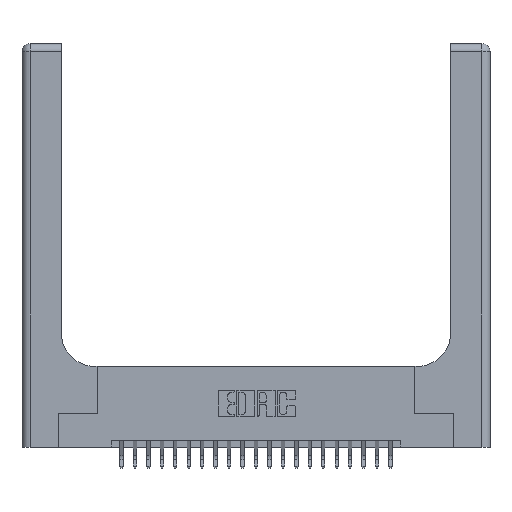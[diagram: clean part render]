
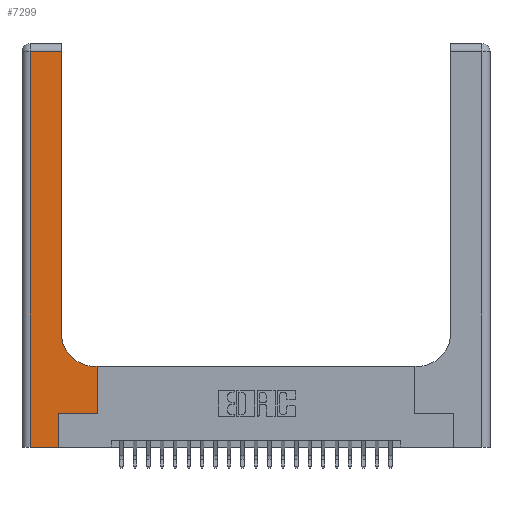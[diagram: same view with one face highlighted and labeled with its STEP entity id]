
A CAD part, top view. The second image highlights one B-rep face of the part: STEP entity #7299.
In plain terms, the highlighted planar face has unit normal (0, 0, 1).
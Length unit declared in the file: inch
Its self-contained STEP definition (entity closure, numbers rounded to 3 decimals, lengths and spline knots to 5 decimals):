
#592 = CARTESIAN_POINT ( 'NONE',  ( 0.269, 0.25, 0.37 ) ) ;
#1023 = VERTEX_POINT ( 'NONE', #11029 ) ;
#1548 = LINE ( 'NONE', #2361, #16248 ) ;
#1916 = VECTOR ( 'NONE', #7862, 39.37008 ) ;
#2361 = CARTESIAN_POINT ( 'NONE',  ( 0.06, 3., 0.37 ) ) ;
#2403 = VECTOR ( 'NONE', #12728, 39.37008 ) ;
#2799 = ORIENTED_EDGE ( 'NONE', *, *, #6019, .T. ) ;
#3022 = EDGE_CURVE ( 'NONE', #11211, #14283, #4676, .T. ) ;
#3046 = LINE ( 'NONE', #18708, #22686 ) ;
#3532 = CARTESIAN_POINT ( 'NONE',  ( 0.5585, 0.25, 0.37 ) ) ;
#3635 = CARTESIAN_POINT ( 'NONE',  ( 0., 3., 0.37 ) ) ;
#4118 = VERTEX_POINT ( 'NONE', #592 ) ;
#4665 = CIRCLE ( 'NONE', #6850, 0.25 ) ;
#4676 = LINE ( 'NONE', #8454, #23669 ) ;
#4746 = ORIENTED_EDGE ( 'NONE', *, *, #21546, .T. ) ;
#4850 = CARTESIAN_POINT ( 'NONE',  ( 0.2915, 2.94, 0.37 ) ) ;
#5420 = VERTEX_POINT ( 'NONE', #18527 ) ;
#5477 = DIRECTION ( 'NONE',  ( 0., 0., -1. ) ) ;
#5487 = DIRECTION ( 'NONE',  ( 0., 1., 0. ) ) ;
#5538 = DIRECTION ( 'NONE',  ( 1., 0., 0. ) ) ;
#5591 = DIRECTION ( 'NONE',  ( 0., 0., -1. ) ) ;
#5747 = VECTOR ( 'NONE', #5538, 39.37008 ) ;
#5763 = LINE ( 'NONE', #3532, #15256 ) ;
#5839 = ORIENTED_EDGE ( 'NONE', *, *, #22563, .T. ) ;
#6015 = FACE_OUTER_BOUND ( 'NONE', #13664, .T. ) ;
#6019 = EDGE_CURVE ( 'NONE', #18812, #18891, #17633, .T. ) ;
#6559 = CARTESIAN_POINT ( 'NONE',  ( 0.2915, 0.85, 0.37 ) ) ;
#6648 = EDGE_CURVE ( 'NONE', #4118, #5420, #10208, .T. ) ;
#6850 = AXIS2_PLACEMENT_3D ( 'NONE', #16830, #5477, #18752 ) ;
#7299 = ADVANCED_FACE ( 'NONE', ( #6015 ), #16934, .F. ) ;
#7862 = DIRECTION ( 'NONE',  ( 1., 0., 0. ) ) ;
#8205 = ORIENTED_EDGE ( 'NONE', *, *, #6648, .T. ) ;
#8454 = CARTESIAN_POINT ( 'NONE',  ( 0.2915, 0.6, 0.37 ) ) ;
#8519 = DIRECTION ( 'NONE',  ( 0., 1., 0. ) ) ;
#8708 = VERTEX_POINT ( 'NONE', #9640 ) ;
#9268 = VECTOR ( 'NONE', #8519, 39.37008 ) ;
#9473 = EDGE_CURVE ( 'NONE', #17769, #4118, #10453, .T. ) ;
#9640 = CARTESIAN_POINT ( 'NONE',  ( 0.06, 0., 0.37 ) ) ;
#10208 = LINE ( 'NONE', #18807, #5747 ) ;
#10453 = LINE ( 'NONE', #21782, #9268 ) ;
#11029 = CARTESIAN_POINT ( 'NONE',  ( 0.06, 2.94, 0.37 ) ) ;
#11211 = VERTEX_POINT ( 'NONE', #21859 ) ;
#11265 = ORIENTED_EDGE ( 'NONE', *, *, #9473, .T. ) ;
#12324 = CARTESIAN_POINT ( 'NONE',  ( 0.269, 0., 0.37 ) ) ;
#12728 = DIRECTION ( 'NONE',  ( 0., 1., 0. ) ) ;
#13084 = DIRECTION ( 'NONE',  ( -1., 0., 0. ) ) ;
#13664 = EDGE_LOOP ( 'NONE', ( #2799, #16541, #21298, #4746, #11265, #8205, #18872, #24474, #5839 ) ) ;
#13856 = DIRECTION ( 'NONE',  ( 0., -1., 0. ) ) ;
#14174 = EDGE_CURVE ( 'NONE', #18891, #1023, #3046, .T. ) ;
#14283 = VERTEX_POINT ( 'NONE', #21269 ) ;
#14622 = CARTESIAN_POINT ( 'NONE',  ( 0.2915, 3., 0.37 ) ) ;
#14730 = EDGE_CURVE ( 'NONE', #5420, #11211, #5763, .T. ) ;
#15256 = VECTOR ( 'NONE', #5487, 39.37008 ) ;
#15473 = CARTESIAN_POINT ( 'NONE',  ( 0., 0., 0.37 ) ) ;
#16248 = VECTOR ( 'NONE', #13856, 39.37008 ) ;
#16541 = ORIENTED_EDGE ( 'NONE', *, *, #14174, .T. ) ;
#16830 = CARTESIAN_POINT ( 'NONE',  ( 0.5415, 0.85, 0.37 ) ) ;
#16934 = PLANE ( 'NONE',  #20056 ) ;
#17633 = LINE ( 'NONE', #14622, #2403 ) ;
#17769 = VERTEX_POINT ( 'NONE', #12324 ) ;
#17786 = LINE ( 'NONE', #15473, #1916 ) ;
#18527 = CARTESIAN_POINT ( 'NONE',  ( 0.5585, 0.25, 0.37 ) ) ;
#18708 = CARTESIAN_POINT ( 'NONE',  ( 0., 2.94, 0.37 ) ) ;
#18752 = DIRECTION ( 'NONE',  ( 1., 0., 0. ) ) ;
#18807 = CARTESIAN_POINT ( 'NONE',  ( 0.269, 0.25, 0.37 ) ) ;
#18812 = VERTEX_POINT ( 'NONE', #6559 ) ;
#18855 = DIRECTION ( 'NONE',  ( -1., 0., 0. ) ) ;
#18872 = ORIENTED_EDGE ( 'NONE', *, *, #14730, .T. ) ;
#18891 = VERTEX_POINT ( 'NONE', #4850 ) ;
#20056 = AXIS2_PLACEMENT_3D ( 'NONE', #3635, #5591, #18855 ) ;
#20499 = EDGE_CURVE ( 'NONE', #1023, #8708, #1548, .T. ) ;
#21269 = CARTESIAN_POINT ( 'NONE',  ( 0.5415, 0.6, 0.37 ) ) ;
#21298 = ORIENTED_EDGE ( 'NONE', *, *, #20499, .T. ) ;
#21546 = EDGE_CURVE ( 'NONE', #8708, #17769, #17786, .T. ) ;
#21711 = DIRECTION ( 'NONE',  ( -1., 0., 0. ) ) ;
#21782 = CARTESIAN_POINT ( 'NONE',  ( 0.269, 0., 0.37 ) ) ;
#21859 = CARTESIAN_POINT ( 'NONE',  ( 0.5585, 0.6, 0.37 ) ) ;
#22563 = EDGE_CURVE ( 'NONE', #14283, #18812, #4665, .T. ) ;
#22686 = VECTOR ( 'NONE', #13084, 39.37008 ) ;
#23669 = VECTOR ( 'NONE', #21711, 39.37008 ) ;
#24474 = ORIENTED_EDGE ( 'NONE', *, *, #3022, .T. ) ;
